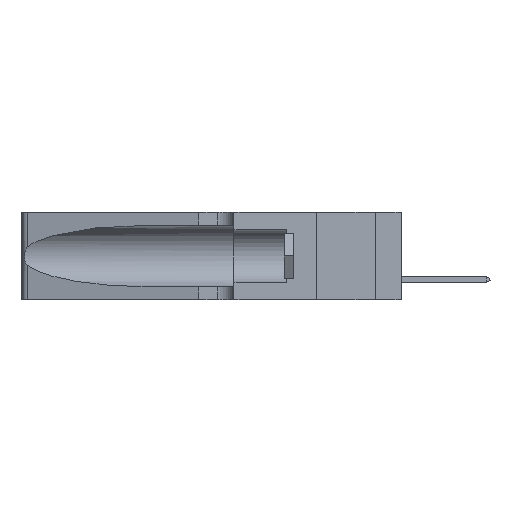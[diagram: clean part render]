
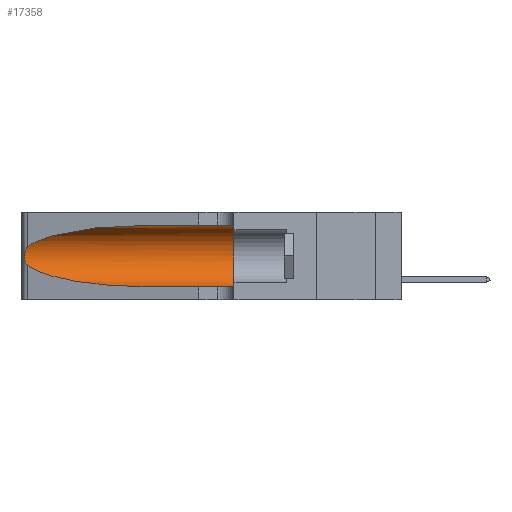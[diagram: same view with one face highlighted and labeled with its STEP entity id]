
A CAD part, left-side view. The second image highlights one B-rep face of the part: STEP entity #17358.
In plain terms, the highlighted cylindrical face has radius 3.308 mm (diameter 6.617 mm), a partial arc.
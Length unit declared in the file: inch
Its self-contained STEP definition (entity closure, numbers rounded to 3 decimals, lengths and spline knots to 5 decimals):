
#129 = B_SPLINE_CURVE_WITH_KNOTS ( 'NONE', 3,
 ( #9919, #29457, #10532, #16363, #19328, #30989, #13567, #1473, #7969, #19950, #5415, #5280, #28464, #16880 ),
 .UNSPECIFIED., .F., .F.,
 ( 4, 2, 2, 2, 2, 2, 4 ),
 ( 0., 0.00027, 0.00053, 0.00107, 0.0016, 0.00187, 0.00214 ),
 .UNSPECIFIED. ) ;
#461 = CARTESIAN_POINT ( 'NONE',  ( 0.1305, 1.61858, 0.31525 ) ) ;
#742 = CARTESIAN_POINT ( 'NONE',  ( 0.1305, 0.72297, 0.31525 ) ) ;
#1473 = CARTESIAN_POINT ( 'NONE',  ( 0.26075, 1.23896, 0.178 ) ) ;
#1742 = VERTEX_POINT ( 'NONE', #20485 ) ;
#2309 = CARTESIAN_POINT ( 'NONE',  ( 0.1305, 0.35, 0.05475 ) ) ;
#2352 = CARTESIAN_POINT ( 'NONE',  ( 0.18966, 0.96281, 0.05475 ) ) ;
#2899 = EDGE_CURVE ( 'NONE', #34308, #33619, #5016, .T. ) ;
#3210 = EDGE_CURVE ( 'NONE', #36249, #1742, #19567, .T. ) ;
#3983 = CARTESIAN_POINT ( 'NONE',  ( 0.25487, 1.22718, 0.14631 ) ) ;
#4017 = EDGE_CURVE ( 'NONE', #12617, #36249, #129, .T. ) ;
#5016 = LINE ( 'NONE', #461, #26831 ) ;
#5280 = CARTESIAN_POINT ( 'NONE',  ( 0.25639, 1.23186, 0.15144 ) ) ;
#5415 = CARTESIAN_POINT ( 'NONE',  ( 0.25789, 1.23486, 0.15765 ) ) ;
#7236 = DIRECTION ( 'NONE',  ( 0., -1., 0. ) ) ;
#7969 = CARTESIAN_POINT ( 'NONE',  ( 0.26017, 1.23833, 0.17102 ) ) ;
#8090 = CARTESIAN_POINT ( 'NONE',  ( 0.1305, 0.72297, 0.05475 ) ) ;
#8334 = DIRECTION ( 'NONE',  ( 0., 0., -1. ) ) ;
#9079 = CARTESIAN_POINT ( 'NONE',  ( 0.1305, 0.72297, 0.31525 ) ) ;
#9552 = DIRECTION ( 'NONE',  ( 0., -1., 0. ) ) ;
#9736 = ORIENTED_EDGE ( 'NONE', *, *, #2899, .F. ) ;
#9919 = CARTESIAN_POINT ( 'NONE',  ( 0.25487, 1.22718, 0.22369 ) ) ;
#9948 = ORIENTED_EDGE ( 'NONE', *, *, #3210, .T. ) ;
#10532 = CARTESIAN_POINT ( 'NONE',  ( 0.25639, 1.23184, 0.21858 ) ) ;
#11026 = CARTESIAN_POINT ( 'NONE',  ( 0.18966, 0.96281, 0.31525 ) ) ;
#11063 = LINE ( 'NONE', #24392, #21005 ) ;
#11646 = CARTESIAN_POINT ( 'NONE',  ( 0.25487, 1.22718, 0.22369 ) ) ;
#11779 = CARTESIAN_POINT ( 'NONE',  ( 0.1305, 0.35, 0.185 ) ) ;
#12617 = VERTEX_POINT ( 'NONE', #11646 ) ;
#12745 =( BOUNDED_CURVE ( )  B_SPLINE_CURVE ( 3, ( #742, #11026, #35456, #17960 ),
 .UNSPECIFIED., .F., .F. ) 
 B_SPLINE_CURVE_WITH_KNOTS ( ( 4, 4 ),
 ( 1.5708, 2.84003 ),
 .UNSPECIFIED. ) 
 CURVE ( )  GEOMETRIC_REPRESENTATION_ITEM ( )  RATIONAL_B_SPLINE_CURVE ( ( 1., 0.87, 0.87, 1. ) ) 
 REPRESENTATION_ITEM ( '' )  );
#13345 = ORIENTED_EDGE ( 'NONE', *, *, #34032, .F. ) ;
#13567 = CARTESIAN_POINT ( 'NONE',  ( 0.26075, 1.23896, 0.19203 ) ) ;
#16047 = AXIS2_PLACEMENT_3D ( 'NONE', #11779, #34666, #20439 ) ;
#16363 = CARTESIAN_POINT ( 'NONE',  ( 0.25787, 1.23484, 0.2124 ) ) ;
#16747 = AXIS2_PLACEMENT_3D ( 'NONE', #34014, #36910, #8334 ) ;
#16880 = CARTESIAN_POINT ( 'NONE',  ( 0.25487, 1.22718, 0.14631 ) ) ;
#17358 = ADVANCED_FACE ( 'NONE', ( #24063 ), #22749, .F. ) ;
#17960 = CARTESIAN_POINT ( 'NONE',  ( 0.25487, 1.22718, 0.22369 ) ) ;
#18660 = CARTESIAN_POINT ( 'NONE',  ( 0.2373, 1.15595, 0.08982 ) ) ;
#19328 = CARTESIAN_POINT ( 'NONE',  ( 0.25854, 1.2359, 0.20912 ) ) ;
#19567 =( BOUNDED_CURVE ( )  B_SPLINE_CURVE ( 3, ( #3983, #18660, #2352, #8090 ),
 .UNSPECIFIED., .F., .F. ) 
 B_SPLINE_CURVE_WITH_KNOTS ( ( 4, 4 ),
 ( 3.44316, 4.71239 ),
 .UNSPECIFIED. ) 
 CURVE ( )  GEOMETRIC_REPRESENTATION_ITEM ( )  RATIONAL_B_SPLINE_CURVE ( ( 1., 0.87, 0.87, 1. ) ) 
 REPRESENTATION_ITEM ( '' )  );
#19950 = CARTESIAN_POINT ( 'NONE',  ( 0.25856, 1.23593, 0.16098 ) ) ;
#20439 = DIRECTION ( 'NONE',  ( 0., 0., 1. ) ) ;
#20485 = CARTESIAN_POINT ( 'NONE',  ( 0.1305, 0.72297, 0.05475 ) ) ;
#20937 = CIRCLE ( 'NONE', #16047, 0.13025 ) ;
#21005 = VECTOR ( 'NONE', #7236, 39.37008 ) ;
#21462 = EDGE_CURVE ( 'NONE', #34308, #12617, #12745, .T. ) ;
#22749 = CYLINDRICAL_SURFACE ( 'NONE', #16747, 0.13025 ) ;
#24063 = FACE_OUTER_BOUND ( 'NONE', #35794, .T. ) ;
#24151 = CARTESIAN_POINT ( 'NONE',  ( 0.1305, 0.35, 0.31525 ) ) ;
#24392 = CARTESIAN_POINT ( 'NONE',  ( 0.1305, 1.61858, 0.05475 ) ) ;
#26672 = ORIENTED_EDGE ( 'NONE', *, *, #33145, .T. ) ;
#26831 = VECTOR ( 'NONE', #9552, 39.37008 ) ;
#28464 = CARTESIAN_POINT ( 'NONE',  ( 0.25555, 1.22993, 0.14849 ) ) ;
#29457 = CARTESIAN_POINT ( 'NONE',  ( 0.25555, 1.22994, 0.2215 ) ) ;
#30845 = ORIENTED_EDGE ( 'NONE', *, *, #4017, .T. ) ;
#30989 = CARTESIAN_POINT ( 'NONE',  ( 0.26018, 1.23835, 0.19895 ) ) ;
#31958 = VERTEX_POINT ( 'NONE', #2309 ) ;
#33145 = EDGE_CURVE ( 'NONE', #1742, #31958, #11063, .T. ) ;
#33306 = CARTESIAN_POINT ( 'NONE',  ( 0.25487, 1.22718, 0.14631 ) ) ;
#33619 = VERTEX_POINT ( 'NONE', #24151 ) ;
#34014 = CARTESIAN_POINT ( 'NONE',  ( 0.1305, 1.61858, 0.185 ) ) ;
#34032 = EDGE_CURVE ( 'NONE', #33619, #31958, #20937, .T. ) ;
#34308 = VERTEX_POINT ( 'NONE', #9079 ) ;
#34666 = DIRECTION ( 'NONE',  ( 0., 1., 0. ) ) ;
#35456 = CARTESIAN_POINT ( 'NONE',  ( 0.2373, 1.15595, 0.28018 ) ) ;
#35745 = ORIENTED_EDGE ( 'NONE', *, *, #21462, .T. ) ;
#35794 = EDGE_LOOP ( 'NONE', ( #35745, #30845, #9948, #26672, #13345, #9736 ) ) ;
#36249 = VERTEX_POINT ( 'NONE', #33306 ) ;
#36910 = DIRECTION ( 'NONE',  ( 0., -1., 0. ) ) ;
